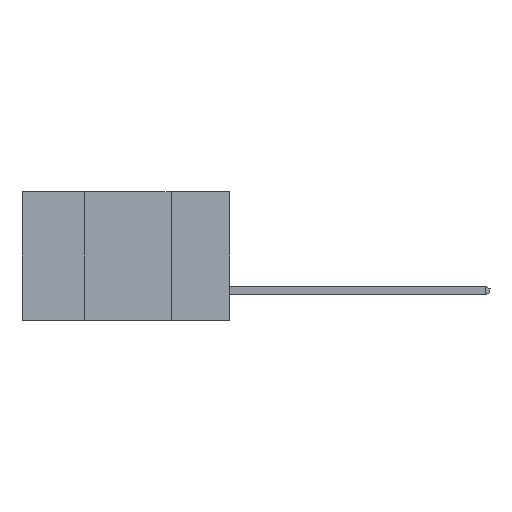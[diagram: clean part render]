
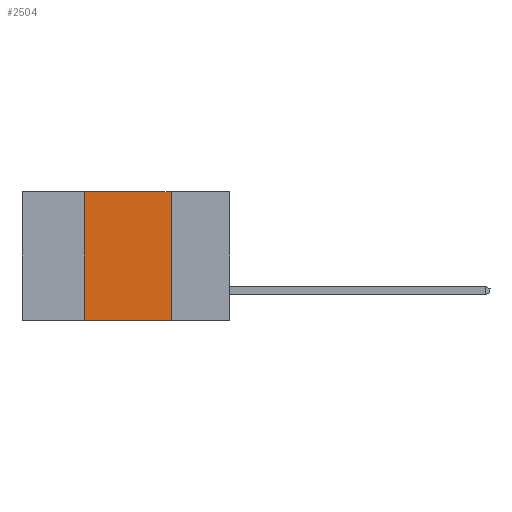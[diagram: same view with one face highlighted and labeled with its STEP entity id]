
A CAD part, left-side view. The second image highlights one B-rep face of the part: STEP entity #2504.
In plain terms, the highlighted planar face has unit normal (-1, 0, 0).
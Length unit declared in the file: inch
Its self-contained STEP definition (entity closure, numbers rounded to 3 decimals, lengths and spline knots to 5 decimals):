
#340 = VECTOR ( 'NONE', #1105, 39.37008 ) ;
#343 = DIRECTION ( 'NONE',  ( 1., 0., 0. ) ) ;
#451 = VECTOR ( 'NONE', #5440, 39.37008 ) ;
#588 = VERTEX_POINT ( 'NONE', #8504 ) ;
#700 = EDGE_CURVE ( 'NONE', #4325, #4920, #3115, .T. ) ;
#1105 = DIRECTION ( 'NONE',  ( 0., -1., 0. ) ) ;
#1143 = CARTESIAN_POINT ( 'NONE',  ( 0., 0.17, -0.37 ) ) ;
#1259 = VERTEX_POINT ( 'NONE', #10540 ) ;
#1278 = LINE ( 'NONE', #1143, #7846 ) ;
#1369 = ORIENTED_EDGE ( 'NONE', *, *, #5511, .F. ) ;
#1724 = CARTESIAN_POINT ( 'NONE',  ( 0., 0.6, 0. ) ) ;
#2504 = ADVANCED_FACE ( 'NONE', ( #5103 ), #10787, .F. ) ;
#2766 = CARTESIAN_POINT ( 'NONE',  ( 0., 0.42, -0.37 ) ) ;
#3115 = LINE ( 'NONE', #6982, #340 ) ;
#3341 = ORIENTED_EDGE ( 'NONE', *, *, #11448, .F. ) ;
#3619 = LINE ( 'NONE', #1724, #451 ) ;
#3663 = AXIS2_PLACEMENT_3D ( 'NONE', #8921, #343, #4162 ) ;
#4162 = DIRECTION ( 'NONE',  ( 0., 0., -1. ) ) ;
#4325 = VERTEX_POINT ( 'NONE', #8100 ) ;
#4511 = EDGE_CURVE ( 'NONE', #4325, #588, #10475, .T. ) ;
#4920 = VERTEX_POINT ( 'NONE', #7389 ) ;
#5103 = FACE_OUTER_BOUND ( 'NONE', #10121, .T. ) ;
#5131 = ORIENTED_EDGE ( 'NONE', *, *, #700, .T. ) ;
#5440 = DIRECTION ( 'NONE',  ( 0., -1., 0. ) ) ;
#5511 = EDGE_CURVE ( 'NONE', #1259, #4920, #1278, .T. ) ;
#6982 = CARTESIAN_POINT ( 'NONE',  ( 0., 0.6, -0.37 ) ) ;
#7389 = CARTESIAN_POINT ( 'NONE',  ( 0., 0.17, -0.37 ) ) ;
#7846 = VECTOR ( 'NONE', #8784, 39.37008 ) ;
#8100 = CARTESIAN_POINT ( 'NONE',  ( 0., 0.42, -0.37 ) ) ;
#8504 = CARTESIAN_POINT ( 'NONE',  ( 0., 0.42, 0. ) ) ;
#8784 = DIRECTION ( 'NONE',  ( 0., 0., -1. ) ) ;
#8921 = CARTESIAN_POINT ( 'NONE',  ( 0., 0.6, 0. ) ) ;
#9815 = ORIENTED_EDGE ( 'NONE', *, *, #4511, .F. ) ;
#10121 = EDGE_LOOP ( 'NONE', ( #1369, #3341, #9815, #5131 ) ) ;
#10168 = VECTOR ( 'NONE', #12261, 39.37008 ) ;
#10475 = LINE ( 'NONE', #2766, #10168 ) ;
#10540 = CARTESIAN_POINT ( 'NONE',  ( 0., 0.17, 0. ) ) ;
#10787 = PLANE ( 'NONE',  #3663 ) ;
#11448 = EDGE_CURVE ( 'NONE', #588, #1259, #3619, .T. ) ;
#12261 = DIRECTION ( 'NONE',  ( 0., 0., 1. ) ) ;
